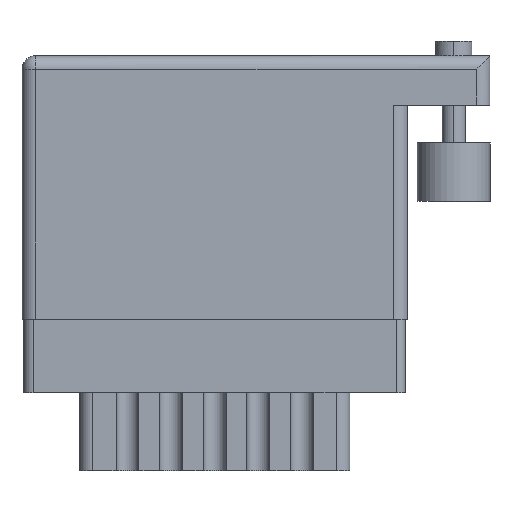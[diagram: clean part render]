
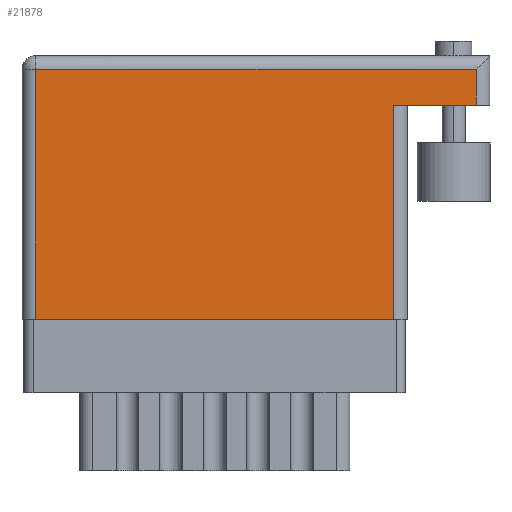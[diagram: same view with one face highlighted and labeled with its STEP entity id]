
A CAD part, front view. The second image highlights one B-rep face of the part: STEP entity #21878.
In plain terms, the highlighted face is planar.
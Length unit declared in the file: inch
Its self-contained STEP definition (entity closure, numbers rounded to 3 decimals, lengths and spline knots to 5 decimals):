
#3 = DIRECTION ( 'NONE',  ( 0., -1., 0. ) ) ;
#2208 = LINE ( 'NONE', #7853, #17948 ) ;
#3440 = VERTEX_POINT ( 'NONE', #23385 ) ;
#4157 = DIRECTION ( 'NONE',  ( -1., 0., 0. ) ) ;
#4282 = EDGE_CURVE ( 'NONE', #6840, #22915, #15744, .T. ) ;
#4513 = EDGE_CURVE ( 'NONE', #18739, #3440, #19333, .T. ) ;
#4595 = CARTESIAN_POINT ( 'NONE',  ( 1.278, 0.736, 0. ) ) ;
#6093 = CARTESIAN_POINT ( 'NONE',  ( 0.047, 0., 0. ) ) ;
#6111 = PLANE ( 'NONE',  #6566 ) ;
#6236 = EDGE_CURVE ( 'NONE', #3440, #12373, #19888, .T. ) ;
#6566 = AXIS2_PLACEMENT_3D ( 'NONE', #14103, #22050, #4157 ) ;
#6840 = VERTEX_POINT ( 'NONE', #9060 ) ;
#7071 = EDGE_CURVE ( 'NONE', #15143, #18739, #2208, .T. ) ;
#7281 = CARTESIAN_POINT ( 'NONE',  ( 1.562, 0.859, 0. ) ) ;
#7578 = LINE ( 'NONE', #15556, #15649 ) ;
#7853 = CARTESIAN_POINT ( 'NONE',  ( 1.562, 0.906, 0. ) ) ;
#9060 = CARTESIAN_POINT ( 'NONE',  ( 1.278, 0., 0. ) ) ;
#10119 = VECTOR ( 'NONE', #19389, 39.37008 ) ;
#10126 = DIRECTION ( 'NONE',  ( -1., 0., 0. ) ) ;
#10354 = VECTOR ( 'NONE', #3, 39.37008 ) ;
#10830 = EDGE_CURVE ( 'NONE', #15143, #22915, #22665, .T. ) ;
#11898 = DIRECTION ( 'NONE',  ( 0., 1., 0. ) ) ;
#12373 = VERTEX_POINT ( 'NONE', #6093 ) ;
#12777 = ORIENTED_EDGE ( 'NONE', *, *, #10830, .F. ) ;
#14103 = CARTESIAN_POINT ( 'NONE',  ( 0., 0.906, 0. ) ) ;
#14494 = CARTESIAN_POINT ( 'NONE',  ( 1.562, 0.736, 0. ) ) ;
#15143 = VERTEX_POINT ( 'NONE', #14494 ) ;
#15556 = CARTESIAN_POINT ( 'NONE',  ( 0., 0., 0. ) ) ;
#15617 = CARTESIAN_POINT ( 'NONE',  ( 1.278, 0.736, 0. ) ) ;
#15649 = VECTOR ( 'NONE', #23511, 39.37008 ) ;
#15744 = LINE ( 'NONE', #15617, #10119 ) ;
#16813 = ORIENTED_EDGE ( 'NONE', *, *, #7071, .T. ) ;
#17938 = CARTESIAN_POINT ( 'NONE',  ( 0.047, 0., 0. ) ) ;
#17948 = VECTOR ( 'NONE', #11898, 39.37008 ) ;
#18013 = FACE_OUTER_BOUND ( 'NONE', #19698, .T. ) ;
#18237 = CARTESIAN_POINT ( 'NONE',  ( 1.609, 0.736, 0. ) ) ;
#18732 = DIRECTION ( 'NONE',  ( -1., 0., 0. ) ) ;
#18739 = VERTEX_POINT ( 'NONE', #7281 ) ;
#19280 = EDGE_CURVE ( 'NONE', #12373, #6840, #7578, .T. ) ;
#19333 = LINE ( 'NONE', #22529, #22245 ) ;
#19389 = DIRECTION ( 'NONE',  ( 0., 1., 0. ) ) ;
#19435 = VECTOR ( 'NONE', #10126, 39.37008 ) ;
#19698 = EDGE_LOOP ( 'NONE', ( #21654, #23877, #12777, #16813, #25044, #22652 ) ) ;
#19888 = LINE ( 'NONE', #17938, #10354 ) ;
#21654 = ORIENTED_EDGE ( 'NONE', *, *, #19280, .T. ) ;
#21878 = ADVANCED_FACE ( 'NONE', ( #18013 ), #6111, .F. ) ;
#22050 = DIRECTION ( 'NONE',  ( 0., 0., -1. ) ) ;
#22245 = VECTOR ( 'NONE', #18732, 39.37008 ) ;
#22529 = CARTESIAN_POINT ( 'NONE',  ( 0., 0.859, 0. ) ) ;
#22652 = ORIENTED_EDGE ( 'NONE', *, *, #6236, .T. ) ;
#22665 = LINE ( 'NONE', #18237, #19435 ) ;
#22915 = VERTEX_POINT ( 'NONE', #4595 ) ;
#23385 = CARTESIAN_POINT ( 'NONE',  ( 0.047, 0.859, 0. ) ) ;
#23511 = DIRECTION ( 'NONE',  ( 1., 0., 0. ) ) ;
#23877 = ORIENTED_EDGE ( 'NONE', *, *, #4282, .T. ) ;
#25044 = ORIENTED_EDGE ( 'NONE', *, *, #4513, .T. ) ;
